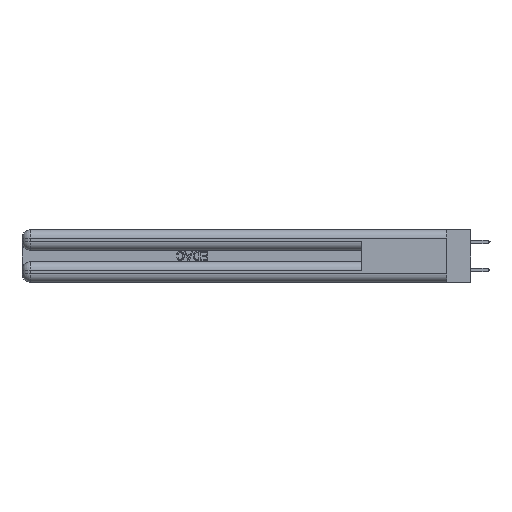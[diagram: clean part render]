
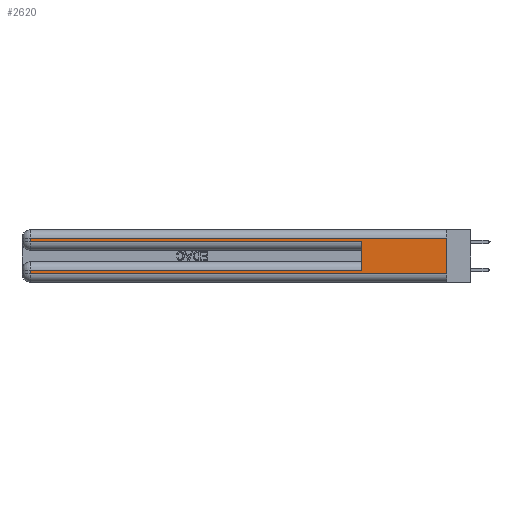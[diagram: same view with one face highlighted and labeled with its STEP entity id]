
A CAD part, left-side view. The second image highlights one B-rep face of the part: STEP entity #2620.
In plain terms, the highlighted planar face has unit normal (-1, 0, 0).
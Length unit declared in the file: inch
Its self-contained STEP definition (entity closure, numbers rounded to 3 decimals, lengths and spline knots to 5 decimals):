
#719 = CARTESIAN_POINT ( 'NONE',  ( 0., 0.6, 0.085 ) ) ;
#1811 = EDGE_CURVE ( 'NONE', #22939, #36515, #38514, .T. ) ;
#2459 = LINE ( 'NONE', #35191, #11565 ) ;
#2620 = ADVANCED_FACE ( 'NONE', ( #21886 ), #11112, .F. ) ;
#2927 = LINE ( 'NONE', #7015, #21209 ) ;
#3511 = VECTOR ( 'NONE', #30853, 39.37008 ) ;
#3940 = VERTEX_POINT ( 'NONE', #13740 ) ;
#4634 = LINE ( 'NONE', #23487, #3511 ) ;
#6109 = VECTOR ( 'NONE', #8568, 39.37008 ) ;
#6214 = CARTESIAN_POINT ( 'NONE',  ( 0., 0., 0.285 ) ) ;
#6705 = DIRECTION ( 'NONE',  ( 0., 1., 0. ) ) ;
#7015 = CARTESIAN_POINT ( 'NONE',  ( 0., 0., 0.085 ) ) ;
#8568 = DIRECTION ( 'NONE',  ( 0., 0., -1. ) ) ;
#9758 = ORIENTED_EDGE ( 'NONE', *, *, #24692, .T. ) ;
#11112 = PLANE ( 'NONE',  #31038 ) ;
#11461 = ORIENTED_EDGE ( 'NONE', *, *, #1811, .T. ) ;
#11565 = VECTOR ( 'NONE', #43702, 39.37008 ) ;
#12176 = VECTOR ( 'NONE', #31808, 39.37008 ) ;
#13374 = ORIENTED_EDGE ( 'NONE', *, *, #34942, .T. ) ;
#13471 = CARTESIAN_POINT ( 'NONE',  ( 0., 2.94, 0.285 ) ) ;
#13740 = CARTESIAN_POINT ( 'NONE',  ( 0., 2.94, 0.31 ) ) ;
#14327 = ORIENTED_EDGE ( 'NONE', *, *, #18190, .T. ) ;
#15071 = EDGE_CURVE ( 'NONE', #17586, #20726, #2459, .T. ) ;
#15773 = LINE ( 'NONE', #30455, #6109 ) ;
#16511 = VECTOR ( 'NONE', #20211, 39.37008 ) ;
#16538 = ORIENTED_EDGE ( 'NONE', *, *, #45035, .F. ) ;
#17586 = VERTEX_POINT ( 'NONE', #30926 ) ;
#18190 = EDGE_CURVE ( 'NONE', #20585, #3940, #33030, .T. ) ;
#18229 = ORIENTED_EDGE ( 'NONE', *, *, #28890, .F. ) ;
#19952 = EDGE_LOOP ( 'NONE', ( #18229, #14327, #9758, #11461, #16538, #27282, #37579, #13374 ) ) ;
#20211 = DIRECTION ( 'NONE',  ( 0., 0., 1. ) ) ;
#20585 = VERTEX_POINT ( 'NONE', #32106 ) ;
#20660 = CARTESIAN_POINT ( 'NONE',  ( 0., 2.94, 0.37 ) ) ;
#20726 = VERTEX_POINT ( 'NONE', #33427 ) ;
#21083 = VECTOR ( 'NONE', #24478, 39.37008 ) ;
#21209 = VECTOR ( 'NONE', #6705, 39.37008 ) ;
#21557 = VECTOR ( 'NONE', #45706, 39.37008 ) ;
#21886 = FACE_OUTER_BOUND ( 'NONE', #19952, .T. ) ;
#22356 = VERTEX_POINT ( 'NONE', #719 ) ;
#22939 = VERTEX_POINT ( 'NONE', #13471 ) ;
#23487 = CARTESIAN_POINT ( 'NONE',  ( 0., 0., 0.06 ) ) ;
#23854 = EDGE_CURVE ( 'NONE', #22356, #17586, #2927, .T. ) ;
#24021 = CARTESIAN_POINT ( 'NONE',  ( 0., 0., 0.06 ) ) ;
#24478 = DIRECTION ( 'NONE',  ( 0., 0., -1. ) ) ;
#24692 = EDGE_CURVE ( 'NONE', #3940, #22939, #41736, .T. ) ;
#26720 = DIRECTION ( 'NONE',  ( 0., 0., -1. ) ) ;
#27282 = ORIENTED_EDGE ( 'NONE', *, *, #23854, .T. ) ;
#28890 = EDGE_CURVE ( 'NONE', #20585, #29644, #15773, .T. ) ;
#29402 = CARTESIAN_POINT ( 'NONE',  ( 0., 0., 0.37 ) ) ;
#29644 = VERTEX_POINT ( 'NONE', #24021 ) ;
#30405 = CARTESIAN_POINT ( 'NONE',  ( 0., 0., 0.31 ) ) ;
#30455 = CARTESIAN_POINT ( 'NONE',  ( 0., 0., 0.37 ) ) ;
#30853 = DIRECTION ( 'NONE',  ( 0., -1., 0. ) ) ;
#30926 = CARTESIAN_POINT ( 'NONE',  ( 0., 2.94, 0.085 ) ) ;
#31038 = AXIS2_PLACEMENT_3D ( 'NONE', #29402, #35375, #26720 ) ;
#31808 = DIRECTION ( 'NONE',  ( 0., -1., 0. ) ) ;
#32106 = CARTESIAN_POINT ( 'NONE',  ( 0., 0., 0.31 ) ) ;
#33030 = LINE ( 'NONE', #30405, #21557 ) ;
#33427 = CARTESIAN_POINT ( 'NONE',  ( 0., 2.94, 0.06 ) ) ;
#34772 = CARTESIAN_POINT ( 'NONE',  ( 0., 0.6, 0.145 ) ) ;
#34942 = EDGE_CURVE ( 'NONE', #20726, #29644, #4634, .T. ) ;
#35191 = CARTESIAN_POINT ( 'NONE',  ( 0., 2.94, 0.37 ) ) ;
#35375 = DIRECTION ( 'NONE',  ( 1., 0., 0. ) ) ;
#36368 = CARTESIAN_POINT ( 'NONE',  ( 0., 0.6, 0.285 ) ) ;
#36515 = VERTEX_POINT ( 'NONE', #36368 ) ;
#37579 = ORIENTED_EDGE ( 'NONE', *, *, #15071, .T. ) ;
#38514 = LINE ( 'NONE', #6214, #12176 ) ;
#41736 = LINE ( 'NONE', #20660, #21083 ) ;
#43702 = DIRECTION ( 'NONE',  ( 0., 0., -1. ) ) ;
#45035 = EDGE_CURVE ( 'NONE', #22356, #36515, #46409, .T. ) ;
#45706 = DIRECTION ( 'NONE',  ( 0., 1., 0. ) ) ;
#46409 = LINE ( 'NONE', #34772, #16511 ) ;
